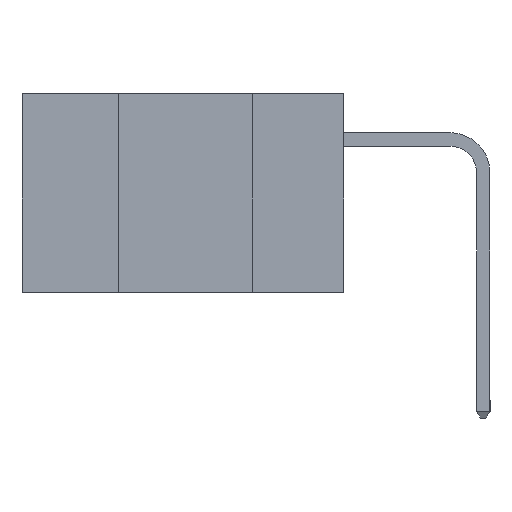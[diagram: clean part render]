
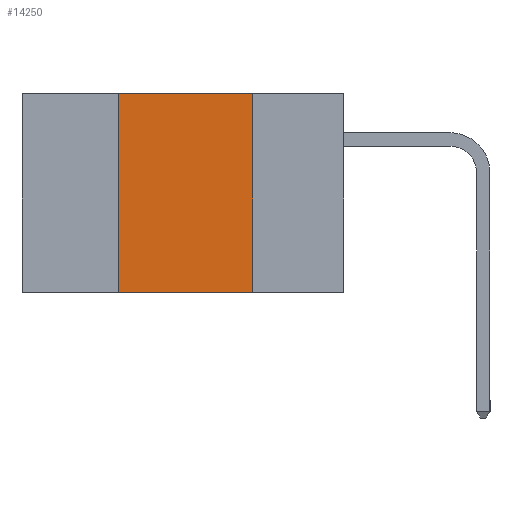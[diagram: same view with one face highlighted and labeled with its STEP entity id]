
A CAD part, left-side view. The second image highlights one B-rep face of the part: STEP entity #14250.
In plain terms, the highlighted planar face has unit normal (-1, 0, 0).
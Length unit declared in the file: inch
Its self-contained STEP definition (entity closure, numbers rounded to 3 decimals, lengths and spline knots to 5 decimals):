
#2 = CARTESIAN_POINT ( 'NONE',  ( 0., 0.17, -0.37 ) ) ;
#38 = DIRECTION ( 'NONE',  ( 1., 0., 0. ) ) ;
#363 = LINE ( 'NONE', #2, #17864 ) ;
#434 = AXIS2_PLACEMENT_3D ( 'NONE', #14058, #38, #10080 ) ;
#1179 = ORIENTED_EDGE ( 'NONE', *, *, #3559, .T. ) ;
#1259 = CARTESIAN_POINT ( 'NONE',  ( 0., 0.17, -0.37 ) ) ;
#1993 = VECTOR ( 'NONE', #2044, 39.37008 ) ;
#2044 = DIRECTION ( 'NONE',  ( 0., 0., 1. ) ) ;
#2370 = ORIENTED_EDGE ( 'NONE', *, *, #11883, .F. ) ;
#2412 = VERTEX_POINT ( 'NONE', #11390 ) ;
#3559 = EDGE_CURVE ( 'NONE', #2412, #9236, #10383, .T. ) ;
#4005 = VERTEX_POINT ( 'NONE', #5088 ) ;
#4532 = EDGE_CURVE ( 'NONE', #2412, #4005, #9521, .T. ) ;
#4656 = DIRECTION ( 'NONE',  ( 0., -1., 0. ) ) ;
#5088 = CARTESIAN_POINT ( 'NONE',  ( 0., 0.42, 0. ) ) ;
#6328 = EDGE_LOOP ( 'NONE', ( #2370, #14658, #12810, #1179 ) ) ;
#6815 = VECTOR ( 'NONE', #11014, 39.37008 ) ;
#8299 = EDGE_CURVE ( 'NONE', #4005, #10730, #16183, .T. ) ;
#8662 = PLANE ( 'NONE',  #434 ) ;
#9236 = VERTEX_POINT ( 'NONE', #1259 ) ;
#9521 = LINE ( 'NONE', #11804, #1993 ) ;
#9988 = DIRECTION ( 'NONE',  ( 0., 0., -1. ) ) ;
#10080 = DIRECTION ( 'NONE',  ( 0., 0., -1. ) ) ;
#10383 = LINE ( 'NONE', #15022, #6815 ) ;
#10730 = VERTEX_POINT ( 'NONE', #15708 ) ;
#11014 = DIRECTION ( 'NONE',  ( 0., -1., 0. ) ) ;
#11390 = CARTESIAN_POINT ( 'NONE',  ( 0., 0.42, -0.37 ) ) ;
#11804 = CARTESIAN_POINT ( 'NONE',  ( 0., 0.42, -0.37 ) ) ;
#11883 = EDGE_CURVE ( 'NONE', #10730, #9236, #363, .T. ) ;
#12065 = FACE_OUTER_BOUND ( 'NONE', #6328, .T. ) ;
#12810 = ORIENTED_EDGE ( 'NONE', *, *, #4532, .F. ) ;
#12837 = CARTESIAN_POINT ( 'NONE',  ( 0., 0.6, 0. ) ) ;
#13047 = VECTOR ( 'NONE', #4656, 39.37008 ) ;
#14058 = CARTESIAN_POINT ( 'NONE',  ( 0., 0.6, 0. ) ) ;
#14250 = ADVANCED_FACE ( 'NONE', ( #12065 ), #8662, .F. ) ;
#14658 = ORIENTED_EDGE ( 'NONE', *, *, #8299, .F. ) ;
#15022 = CARTESIAN_POINT ( 'NONE',  ( 0., 0.6, -0.37 ) ) ;
#15708 = CARTESIAN_POINT ( 'NONE',  ( 0., 0.17, 0. ) ) ;
#16183 = LINE ( 'NONE', #12837, #13047 ) ;
#17864 = VECTOR ( 'NONE', #9988, 39.37008 ) ;
